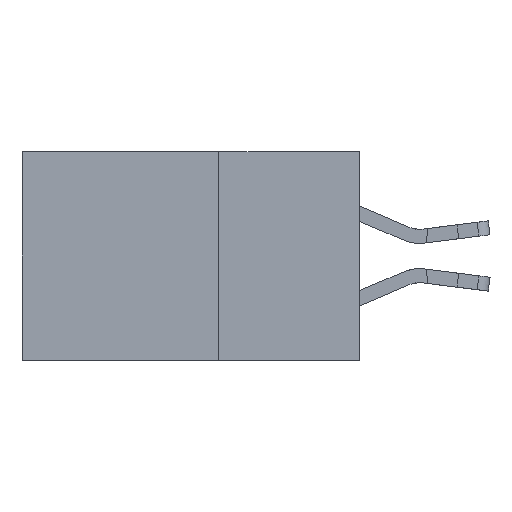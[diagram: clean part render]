
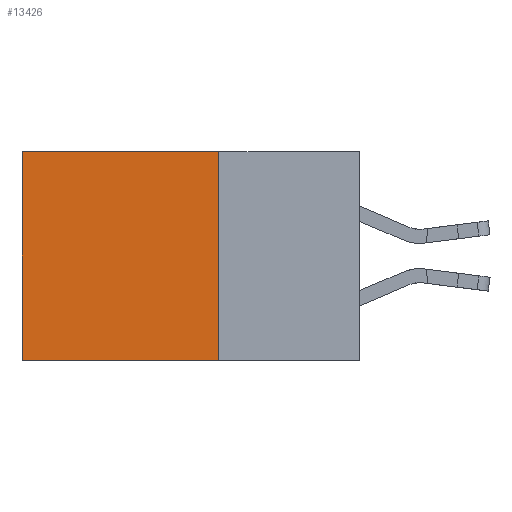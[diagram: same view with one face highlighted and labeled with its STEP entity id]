
A CAD part, left-side view. The second image highlights one B-rep face of the part: STEP entity #13426.
In plain terms, the highlighted planar face has unit normal (-1, 0, 0).
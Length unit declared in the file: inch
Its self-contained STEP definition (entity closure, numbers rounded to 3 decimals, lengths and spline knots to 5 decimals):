
#96 = AXIS2_PLACEMENT_3D ( 'NONE', #15991, #5011, #17922 ) ;
#283 = VECTOR ( 'NONE', #643, 39.37008 ) ;
#643 = DIRECTION ( 'NONE',  ( 0., 1., 0. ) ) ;
#1022 = ORIENTED_EDGE ( 'NONE', *, *, #22773, .T. ) ;
#1475 = LINE ( 'NONE', #4238, #20607 ) ;
#2241 = VECTOR ( 'NONE', #12212, 39.37008 ) ;
#4238 = CARTESIAN_POINT ( 'NONE',  ( 0.2875, 0.25, -0.37 ) ) ;
#5011 = DIRECTION ( 'NONE',  ( 1., 0., 0. ) ) ;
#5012 = EDGE_CURVE ( 'NONE', #15703, #20486, #22000, .T. ) ;
#5583 = CARTESIAN_POINT ( 'NONE',  ( 0.2875, 0.6, -0.37 ) ) ;
#6109 = CARTESIAN_POINT ( 'NONE',  ( 0.2875, 0.25, 0. ) ) ;
#7031 = ORIENTED_EDGE ( 'NONE', *, *, #5012, .F. ) ;
#7297 = VECTOR ( 'NONE', #21722, 39.37008 ) ;
#8845 = CARTESIAN_POINT ( 'NONE',  ( 0.2875, 0.25, 0. ) ) ;
#11341 = FACE_OUTER_BOUND ( 'NONE', #22255, .T. ) ;
#11351 = ORIENTED_EDGE ( 'NONE', *, *, #11429, .T. ) ;
#11429 = EDGE_CURVE ( 'NONE', #15703, #13822, #19420, .T. ) ;
#11849 = CARTESIAN_POINT ( 'NONE',  ( 0.2875, 0.25, 0. ) ) ;
#12212 = DIRECTION ( 'NONE',  ( 0., 0., -1. ) ) ;
#13329 = LINE ( 'NONE', #21345, #2241 ) ;
#13426 = ADVANCED_FACE ( 'NONE', ( #11341 ), #16069, .F. ) ;
#13822 = VERTEX_POINT ( 'NONE', #22800 ) ;
#14874 = VERTEX_POINT ( 'NONE', #5583 ) ;
#15703 = VERTEX_POINT ( 'NONE', #6109 ) ;
#15991 = CARTESIAN_POINT ( 'NONE',  ( 0.2875, 0.25, 0. ) ) ;
#16031 = CARTESIAN_POINT ( 'NONE',  ( 0.2875, 0.25, -0.37 ) ) ;
#16069 = PLANE ( 'NONE',  #96 ) ;
#17922 = DIRECTION ( 'NONE',  ( 0., 0., -1. ) ) ;
#19420 = LINE ( 'NONE', #11849, #283 ) ;
#20268 = EDGE_CURVE ( 'NONE', #20486, #14874, #1475, .T. ) ;
#20486 = VERTEX_POINT ( 'NONE', #16031 ) ;
#20607 = VECTOR ( 'NONE', #20894, 39.37008 ) ;
#20723 = ORIENTED_EDGE ( 'NONE', *, *, #20268, .F. ) ;
#20894 = DIRECTION ( 'NONE',  ( 0., 1., 0. ) ) ;
#21345 = CARTESIAN_POINT ( 'NONE',  ( 0.2875, 0.6, 0. ) ) ;
#21722 = DIRECTION ( 'NONE',  ( 0., 0., -1. ) ) ;
#22000 = LINE ( 'NONE', #8845, #7297 ) ;
#22255 = EDGE_LOOP ( 'NONE', ( #1022, #20723, #7031, #11351 ) ) ;
#22773 = EDGE_CURVE ( 'NONE', #13822, #14874, #13329, .T. ) ;
#22800 = CARTESIAN_POINT ( 'NONE',  ( 0.2875, 0.6, 0. ) ) ;
